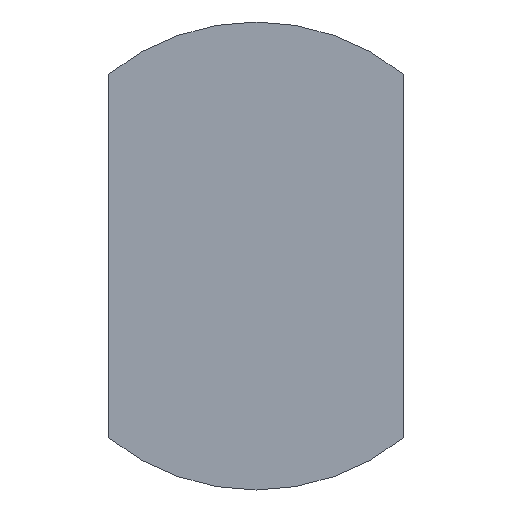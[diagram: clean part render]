
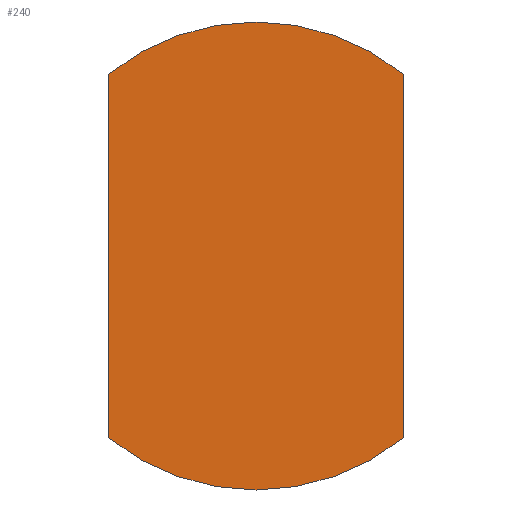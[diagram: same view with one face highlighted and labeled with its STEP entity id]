
A CAD part, front view. The second image highlights one B-rep face of the part: STEP entity #240.
In plain terms, the highlighted planar face has unit normal (0, -1, 0).
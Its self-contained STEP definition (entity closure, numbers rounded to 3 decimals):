
#62=DIRECTION('',(0.,0.,-1.));
#63=VECTOR('',#62,7.766);
#64=CARTESIAN_POINT('',(3.15,-3.,3.883));
#65=LINE('',#64,#63);
#66=CARTESIAN_POINT('',(0.,-3.,0.));
#67=DIRECTION('',(0.,1.,0.));
#68=DIRECTION('',(0.63,0.,-0.777));
#69=AXIS2_PLACEMENT_3D('',#66,#67,#68);
#71=DIRECTION('',(0.,0.,1.));
#72=VECTOR('',#71,7.766);
#73=CARTESIAN_POINT('',(-3.15,-3.,-3.883));
#74=LINE('',#73,#72);
#75=CARTESIAN_POINT('',(0.,-3.,0.));
#76=DIRECTION('',(0.,1.,0.));
#77=DIRECTION('',(-0.63,0.,0.777));
#78=AXIS2_PLACEMENT_3D('',#75,#76,#77);
#101=CARTESIAN_POINT('',(3.15,-3.,3.883));
#102=CARTESIAN_POINT('',(3.15,-3.,-3.883));
#103=VERTEX_POINT('',#101);
#104=VERTEX_POINT('',#102);
#109=CARTESIAN_POINT('',(-3.15,-3.,-3.883));
#110=VERTEX_POINT('',#109);
#111=CARTESIAN_POINT('',(-3.15,-3.,3.883));
#112=VERTEX_POINT('',#111);
#229=CARTESIAN_POINT('',(0.,-3.,0.));
#230=DIRECTION('',(0.,1.,0.));
#231=DIRECTION('',(1.,0.,0.));
#232=AXIS2_PLACEMENT_3D('',#229,#230,#231);
#233=PLANE('',#232);
#234=ORIENTED_EDGE('',*,*,#180,.T.);
#235=ORIENTED_EDGE('',*,*,#196,.T.);
#236=ORIENTED_EDGE('',*,*,#210,.T.);
#237=ORIENTED_EDGE('',*,*,#222,.T.);
#238=EDGE_LOOP('',(#234,#235,#236,#237));
#239=FACE_OUTER_BOUND('',#238,.F.);
#240=ADVANCED_FACE('',(#239),#233,.F.);
#70=CIRCLE('',#69,5.);
#79=CIRCLE('',#78,5.);
#180=EDGE_CURVE('',#103,#104,#65,.T.);
#196=EDGE_CURVE('',#104,#110,#70,.T.);
#210=EDGE_CURVE('',#110,#112,#74,.T.);
#222=EDGE_CURVE('',#112,#103,#79,.T.);
